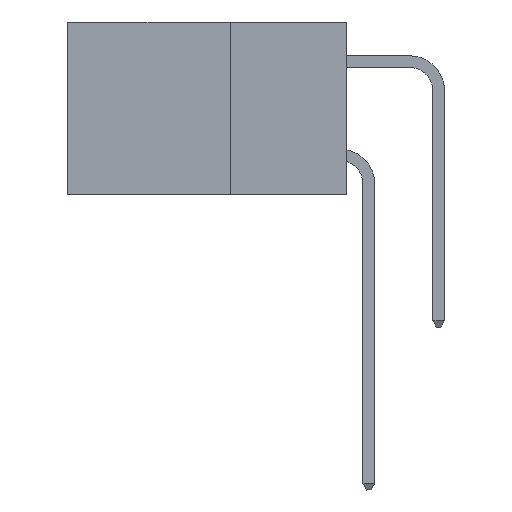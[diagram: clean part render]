
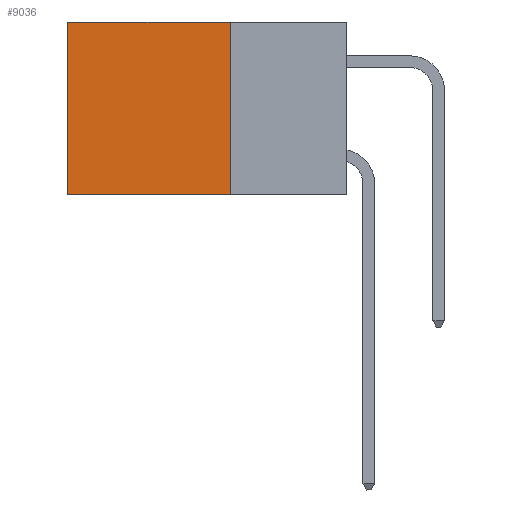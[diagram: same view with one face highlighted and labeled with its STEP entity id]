
A CAD part, left-side view. The second image highlights one B-rep face of the part: STEP entity #9036.
In plain terms, the highlighted planar face has unit normal (-1, 0, 0).
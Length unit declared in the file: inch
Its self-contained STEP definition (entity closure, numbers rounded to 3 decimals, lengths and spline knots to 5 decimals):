
#494 = CARTESIAN_POINT ( 'NONE',  ( 0.2875, 0.6, 0. ) ) ;
#677 = DIRECTION ( 'NONE',  ( 0., 0., -1. ) ) ;
#1082 = VECTOR ( 'NONE', #10649, 39.37008 ) ;
#1204 = EDGE_CURVE ( 'NONE', #9666, #16306, #9392, .T. ) ;
#1611 = VECTOR ( 'NONE', #677, 39.37008 ) ;
#1787 = EDGE_LOOP ( 'NONE', ( #8790, #16913, #17975, #10451 ) ) ;
#2647 = CARTESIAN_POINT ( 'NONE',  ( 0.2875, 0.25, 0. ) ) ;
#2836 = CARTESIAN_POINT ( 'NONE',  ( 0.2875, 0.25, -0.37 ) ) ;
#3515 = PLANE ( 'NONE',  #5962 ) ;
#3939 = EDGE_CURVE ( 'NONE', #4592, #9478, #12491, .T. ) ;
#4560 = CARTESIAN_POINT ( 'NONE',  ( 0.2875, 0.6, -0.37 ) ) ;
#4592 = VERTEX_POINT ( 'NONE', #14890 ) ;
#5962 = AXIS2_PLACEMENT_3D ( 'NONE', #14737, #6511, #16119 ) ;
#6511 = DIRECTION ( 'NONE',  ( 1., 0., 0. ) ) ;
#7096 = VECTOR ( 'NONE', #14372, 39.37008 ) ;
#7371 = VECTOR ( 'NONE', #11287, 39.37008 ) ;
#7436 = CARTESIAN_POINT ( 'NONE',  ( 0.2875, 0.25, 0. ) ) ;
#8790 = ORIENTED_EDGE ( 'NONE', *, *, #3939, .T. ) ;
#9036 = ADVANCED_FACE ( 'NONE', ( #13264 ), #3515, .F. ) ;
#9392 = LINE ( 'NONE', #7436, #1611 ) ;
#9478 = VERTEX_POINT ( 'NONE', #4560 ) ;
#9666 = VERTEX_POINT ( 'NONE', #16098 ) ;
#10451 = ORIENTED_EDGE ( 'NONE', *, *, #13226, .T. ) ;
#10649 = DIRECTION ( 'NONE',  ( 0., 0., -1. ) ) ;
#11287 = DIRECTION ( 'NONE',  ( 0., 1., 0. ) ) ;
#12491 = LINE ( 'NONE', #494, #1082 ) ;
#13226 = EDGE_CURVE ( 'NONE', #9666, #4592, #14625, .T. ) ;
#13264 = FACE_OUTER_BOUND ( 'NONE', #1787, .T. ) ;
#14372 = DIRECTION ( 'NONE',  ( 0., 1., 0. ) ) ;
#14430 = EDGE_CURVE ( 'NONE', #16306, #9478, #17972, .T. ) ;
#14625 = LINE ( 'NONE', #2647, #7371 ) ;
#14737 = CARTESIAN_POINT ( 'NONE',  ( 0.2875, 0.25, 0. ) ) ;
#14890 = CARTESIAN_POINT ( 'NONE',  ( 0.2875, 0.6, 0. ) ) ;
#16098 = CARTESIAN_POINT ( 'NONE',  ( 0.2875, 0.25, 0. ) ) ;
#16119 = DIRECTION ( 'NONE',  ( 0., 0., -1. ) ) ;
#16306 = VERTEX_POINT ( 'NONE', #2836 ) ;
#16913 = ORIENTED_EDGE ( 'NONE', *, *, #14430, .F. ) ;
#17103 = CARTESIAN_POINT ( 'NONE',  ( 0.2875, 0.25, -0.37 ) ) ;
#17972 = LINE ( 'NONE', #17103, #7096 ) ;
#17975 = ORIENTED_EDGE ( 'NONE', *, *, #1204, .F. ) ;
